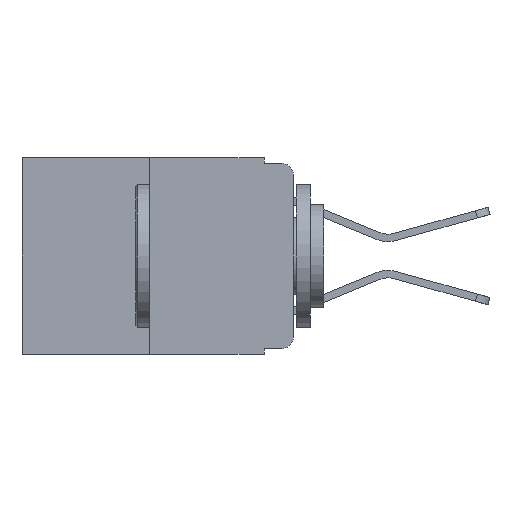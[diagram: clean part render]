
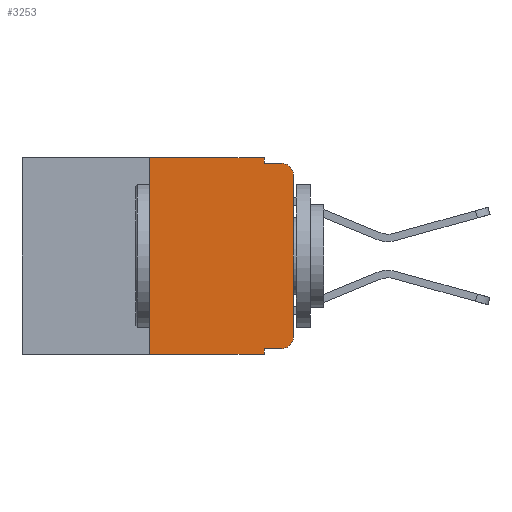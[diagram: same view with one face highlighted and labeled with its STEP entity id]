
A CAD part, left-side view. The second image highlights one B-rep face of the part: STEP entity #3253.
In plain terms, the highlighted planar face has unit normal (-1, 0, 0).
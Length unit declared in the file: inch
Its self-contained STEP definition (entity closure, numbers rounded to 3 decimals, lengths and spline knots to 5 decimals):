
#342 = CARTESIAN_POINT ( 'NONE',  ( 0., 0.051, 0. ) ) ;
#395 = CARTESIAN_POINT ( 'NONE',  ( 0., 0.051, -0.333 ) ) ;
#602 = DIRECTION ( 'NONE',  ( 0., -1., 0. ) ) ;
#691 = ORIENTED_EDGE ( 'NONE', *, *, #10491, .T. ) ;
#884 = EDGE_CURVE ( 'NONE', #3688, #10306, #11834, .T. ) ;
#1194 = CIRCLE ( 'NONE', #6041, 0.02 ) ;
#1369 = DIRECTION ( 'NONE',  ( 0., 0., -1. ) ) ;
#1530 = CARTESIAN_POINT ( 'NONE',  ( 0., 0.051, 0. ) ) ;
#1545 = DIRECTION ( 'NONE',  ( 0., 0., -1. ) ) ;
#1604 = CARTESIAN_POINT ( 'NONE',  ( 0., 0.473, 0. ) ) ;
#1676 = EDGE_CURVE ( 'NONE', #1848, #3688, #11322, .T. ) ;
#1848 = VERTEX_POINT ( 'NONE', #395 ) ;
#1902 = CARTESIAN_POINT ( 'NONE',  ( 0., 0.051, -0.01 ) ) ;
#1974 = CARTESIAN_POINT ( 'NONE',  ( 0., 0.25, 0. ) ) ;
#2179 = VERTEX_POINT ( 'NONE', #7072 ) ;
#2330 = VERTEX_POINT ( 'NONE', #4999 ) ;
#2621 = VECTOR ( 'NONE', #1369, 39.37008 ) ;
#2671 = CARTESIAN_POINT ( 'NONE',  ( 0., 0.02, -0.03 ) ) ;
#2829 = FACE_OUTER_BOUND ( 'NONE', #12207, .T. ) ;
#3253 = ADVANCED_FACE ( 'NONE', ( #2829 ), #5671, .F. ) ;
#3456 = ORIENTED_EDGE ( 'NONE', *, *, #5327, .F. ) ;
#3511 = CARTESIAN_POINT ( 'NONE',  ( 0., 0.051, -0.01 ) ) ;
#3688 = VERTEX_POINT ( 'NONE', #14106 ) ;
#3736 = EDGE_CURVE ( 'NONE', #10306, #6112, #11282, .T. ) ;
#3860 = DIRECTION ( 'NONE',  ( 0., 0., -1. ) ) ;
#4016 = LINE ( 'NONE', #1604, #12681 ) ;
#4032 = VECTOR ( 'NONE', #4302, 39.37008 ) ;
#4043 = EDGE_CURVE ( 'NONE', #1848, #10764, #10775, .T. ) ;
#4208 = ORIENTED_EDGE ( 'NONE', *, *, #4043, .F. ) ;
#4302 = DIRECTION ( 'NONE',  ( 0., 0., 1. ) ) ;
#4496 = CARTESIAN_POINT ( 'NONE',  ( 0., 0., 0. ) ) ;
#4813 = EDGE_CURVE ( 'NONE', #2179, #6580, #9903, .T. ) ;
#4999 = CARTESIAN_POINT ( 'NONE',  ( 0., 0.02, -0.01 ) ) ;
#5233 = DIRECTION ( 'NONE',  ( 0., 0., 1. ) ) ;
#5327 = EDGE_CURVE ( 'NONE', #6580, #14311, #4016, .T. ) ;
#5332 = CARTESIAN_POINT ( 'NONE',  ( 0., 0.473, -0.343 ) ) ;
#5432 = DIRECTION ( 'NONE',  ( 0., -1., 0. ) ) ;
#5671 = PLANE ( 'NONE',  #7290 ) ;
#6041 = AXIS2_PLACEMENT_3D ( 'NONE', #2671, #10443, #3860 ) ;
#6112 = VERTEX_POINT ( 'NONE', #13250 ) ;
#6139 = VERTEX_POINT ( 'NONE', #3511 ) ;
#6483 = DIRECTION ( 'NONE',  ( 1., 0., 0. ) ) ;
#6580 = VERTEX_POINT ( 'NONE', #1974 ) ;
#6595 = DIRECTION ( 'NONE',  ( 0., 0., -1. ) ) ;
#7072 = CARTESIAN_POINT ( 'NONE',  ( 0., 0.25, -0.343 ) ) ;
#7086 = EDGE_CURVE ( 'NONE', #14311, #6139, #10679, .T. ) ;
#7209 = ORIENTED_EDGE ( 'NONE', *, *, #1676, .T. ) ;
#7290 = AXIS2_PLACEMENT_3D ( 'NONE', #10453, #6483, #9249 ) ;
#7795 = EDGE_CURVE ( 'NONE', #6139, #2330, #12802, .T. ) ;
#7848 = DIRECTION ( 'NONE',  ( 0., -1., 0. ) ) ;
#8356 = ORIENTED_EDGE ( 'NONE', *, *, #3736, .T. ) ;
#8508 = VECTOR ( 'NONE', #7848, 39.37008 ) ;
#8519 = EDGE_CURVE ( 'NONE', #6112, #2330, #1194, .T. ) ;
#8599 = LINE ( 'NONE', #5332, #13880 ) ;
#9249 = DIRECTION ( 'NONE',  ( 0., 0., -1. ) ) ;
#9903 = LINE ( 'NONE', #12899, #4032 ) ;
#10012 = VECTOR ( 'NONE', #5432, 39.37008 ) ;
#10041 = ORIENTED_EDGE ( 'NONE', *, *, #884, .T. ) ;
#10306 = VERTEX_POINT ( 'NONE', #10495 ) ;
#10336 = CARTESIAN_POINT ( 'NONE',  ( 0., 0.051, 0. ) ) ;
#10443 = DIRECTION ( 'NONE',  ( -1., 0., 0. ) ) ;
#10453 = CARTESIAN_POINT ( 'NONE',  ( 0., 0.473, 0. ) ) ;
#10491 = EDGE_CURVE ( 'NONE', #2179, #10764, #8599, .T. ) ;
#10495 = CARTESIAN_POINT ( 'NONE',  ( 0., 0., -0.313 ) ) ;
#10679 = LINE ( 'NONE', #342, #12474 ) ;
#10764 = VERTEX_POINT ( 'NONE', #12264 ) ;
#10775 = LINE ( 'NONE', #1530, #2621 ) ;
#10955 = VECTOR ( 'NONE', #5233, 39.37008 ) ;
#11282 = LINE ( 'NONE', #4496, #10955 ) ;
#11322 = LINE ( 'NONE', #13141, #8508 ) ;
#11519 = ORIENTED_EDGE ( 'NONE', *, *, #7795, .F. ) ;
#11590 = DIRECTION ( 'NONE',  ( 0., -1., 0. ) ) ;
#11834 = CIRCLE ( 'NONE', #14360, 0.02 ) ;
#11845 = ORIENTED_EDGE ( 'NONE', *, *, #7086, .F. ) ;
#12172 = ORIENTED_EDGE ( 'NONE', *, *, #4813, .F. ) ;
#12194 = CARTESIAN_POINT ( 'NONE',  ( 0., 0.02, -0.313 ) ) ;
#12207 = EDGE_LOOP ( 'NONE', ( #8356, #13990, #11519, #11845, #3456, #12172, #691, #4208, #7209, #10041 ) ) ;
#12264 = CARTESIAN_POINT ( 'NONE',  ( 0., 0.051, -0.343 ) ) ;
#12474 = VECTOR ( 'NONE', #1545, 39.37008 ) ;
#12681 = VECTOR ( 'NONE', #11590, 39.37008 ) ;
#12802 = LINE ( 'NONE', #1902, #10012 ) ;
#12899 = CARTESIAN_POINT ( 'NONE',  ( 0., 0.25, 0. ) ) ;
#13141 = CARTESIAN_POINT ( 'NONE',  ( 0., 0.051, -0.333 ) ) ;
#13250 = CARTESIAN_POINT ( 'NONE',  ( 0., 0., -0.03 ) ) ;
#13866 = DIRECTION ( 'NONE',  ( -1., 0., 0. ) ) ;
#13880 = VECTOR ( 'NONE', #602, 39.37008 ) ;
#13990 = ORIENTED_EDGE ( 'NONE', *, *, #8519, .T. ) ;
#14106 = CARTESIAN_POINT ( 'NONE',  ( 0., 0.02, -0.333 ) ) ;
#14311 = VERTEX_POINT ( 'NONE', #10336 ) ;
#14360 = AXIS2_PLACEMENT_3D ( 'NONE', #12194, #13866, #6595 ) ;
